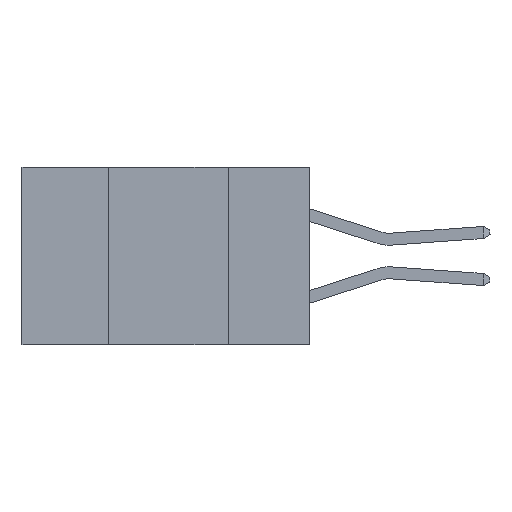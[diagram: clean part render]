
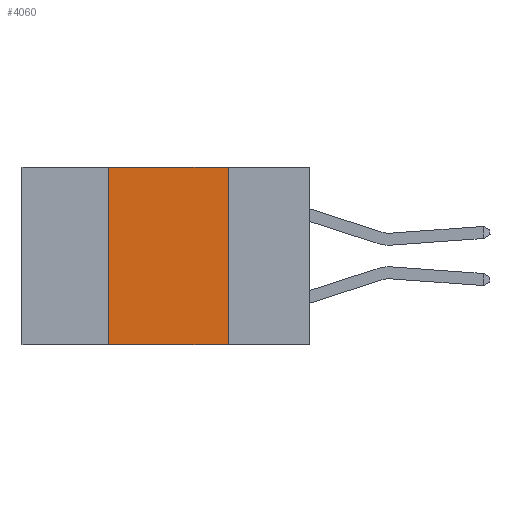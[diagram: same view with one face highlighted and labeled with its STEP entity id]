
A CAD part, left-side view. The second image highlights one B-rep face of the part: STEP entity #4060.
In plain terms, the highlighted planar face has unit normal (-1, 0, 0).
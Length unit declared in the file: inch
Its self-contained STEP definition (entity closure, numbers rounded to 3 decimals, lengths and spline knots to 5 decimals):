
#303 = CARTESIAN_POINT ( 'NONE',  ( 0., 0.42, 0. ) ) ;
#630 = DIRECTION ( 'NONE',  ( 0., -1., 0. ) ) ;
#640 = VERTEX_POINT ( 'NONE', #4978 ) ;
#947 = LINE ( 'NONE', #11496, #4466 ) ;
#1034 = VERTEX_POINT ( 'NONE', #8732 ) ;
#1761 = EDGE_CURVE ( 'NONE', #1034, #640, #7108, .T. ) ;
#2001 = ORIENTED_EDGE ( 'NONE', *, *, #8803, .F. ) ;
#2170 = DIRECTION ( 'NONE',  ( 0., 0., 1. ) ) ;
#2209 = CARTESIAN_POINT ( 'NONE',  ( 0., 0.17, 0. ) ) ;
#2291 = DIRECTION ( 'NONE',  ( 0., 0., -1. ) ) ;
#3487 = CARTESIAN_POINT ( 'NONE',  ( 0., 0.17, -0.37 ) ) ;
#3641 = LINE ( 'NONE', #303, #8989 ) ;
#4060 = ADVANCED_FACE ( 'NONE', ( #9791 ), #12592, .F. ) ;
#4064 = CARTESIAN_POINT ( 'NONE',  ( 0., 0.42, -0.37 ) ) ;
#4439 = VECTOR ( 'NONE', #2291, 39.37008 ) ;
#4441 = EDGE_CURVE ( 'NONE', #640, #7275, #9616, .T. ) ;
#4466 = VECTOR ( 'NONE', #5691, 39.37008 ) ;
#4500 = VECTOR ( 'NONE', #630, 39.37008 ) ;
#4978 = CARTESIAN_POINT ( 'NONE',  ( 0., 0.17, 0. ) ) ;
#5479 = EDGE_LOOP ( 'NONE', ( #8462, #10435, #2001, #10217 ) ) ;
#5635 = CARTESIAN_POINT ( 'NONE',  ( 0., 0.6, 0. ) ) ;
#5691 = DIRECTION ( 'NONE',  ( 0., -1., 0. ) ) ;
#6274 = AXIS2_PLACEMENT_3D ( 'NONE', #5635, #8548, #7595 ) ;
#7108 = LINE ( 'NONE', #7308, #4500 ) ;
#7275 = VERTEX_POINT ( 'NONE', #3487 ) ;
#7308 = CARTESIAN_POINT ( 'NONE',  ( 0., 0.6, 0. ) ) ;
#7362 = EDGE_CURVE ( 'NONE', #12526, #7275, #947, .T. ) ;
#7595 = DIRECTION ( 'NONE',  ( 0., 0., -1. ) ) ;
#8462 = ORIENTED_EDGE ( 'NONE', *, *, #4441, .F. ) ;
#8548 = DIRECTION ( 'NONE',  ( 1., 0., 0. ) ) ;
#8732 = CARTESIAN_POINT ( 'NONE',  ( 0., 0.42, 0. ) ) ;
#8803 = EDGE_CURVE ( 'NONE', #12526, #1034, #3641, .T. ) ;
#8989 = VECTOR ( 'NONE', #2170, 39.37008 ) ;
#9616 = LINE ( 'NONE', #2209, #4439 ) ;
#9791 = FACE_OUTER_BOUND ( 'NONE', #5479, .T. ) ;
#10217 = ORIENTED_EDGE ( 'NONE', *, *, #7362, .T. ) ;
#10435 = ORIENTED_EDGE ( 'NONE', *, *, #1761, .F. ) ;
#11496 = CARTESIAN_POINT ( 'NONE',  ( 0., 0.6, -0.37 ) ) ;
#12526 = VERTEX_POINT ( 'NONE', #4064 ) ;
#12592 = PLANE ( 'NONE',  #6274 ) ;
